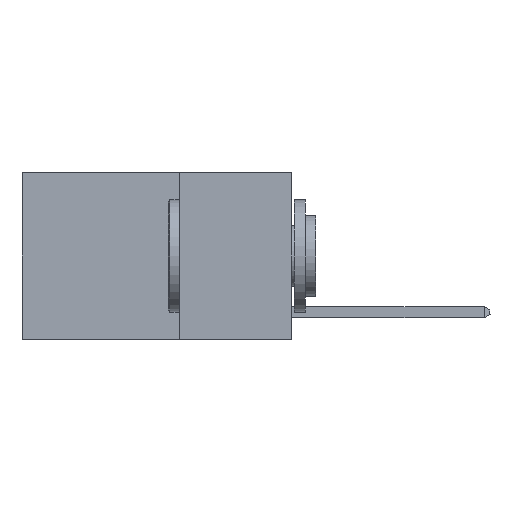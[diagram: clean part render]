
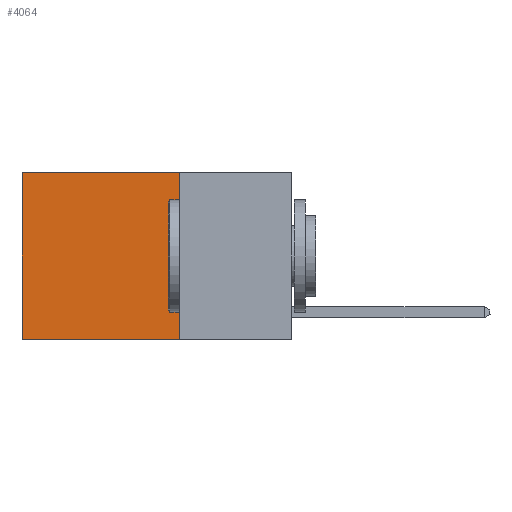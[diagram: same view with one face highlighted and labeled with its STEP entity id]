
A CAD part, left-side view. The second image highlights one B-rep face of the part: STEP entity #4064.
In plain terms, the highlighted planar face has unit normal (-1, 0, 0).
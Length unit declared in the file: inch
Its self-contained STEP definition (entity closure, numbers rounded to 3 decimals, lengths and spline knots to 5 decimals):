
#408 = AXIS2_PLACEMENT_3D ( 'NONE', #5421, #14235, #3438 ) ;
#579 = VECTOR ( 'NONE', #27081, 39.37008 ) ;
#3438 = DIRECTION ( 'NONE',  ( 0., 0., -1. ) ) ;
#3448 = CARTESIAN_POINT ( 'NONE',  ( 0.2625, 0.25, 0. ) ) ;
#3665 = EDGE_CURVE ( 'NONE', #5362, #18175, #24230, .T. ) ;
#4064 = ADVANCED_FACE ( 'NONE', ( #27777 ), #16918, .F. ) ;
#4445 = CARTESIAN_POINT ( 'NONE',  ( 0.2625, 0.25, 0. ) ) ;
#5362 = VERTEX_POINT ( 'NONE', #3448 ) ;
#5421 = CARTESIAN_POINT ( 'NONE',  ( 0.2625, 0.25, 0. ) ) ;
#7192 = ORIENTED_EDGE ( 'NONE', *, *, #16815, .T. ) ;
#8662 = DIRECTION ( 'NONE',  ( 0., 0., -1. ) ) ;
#9347 = CARTESIAN_POINT ( 'NONE',  ( 0.2625, 0.6, 0. ) ) ;
#9822 = LINE ( 'NONE', #24672, #24965 ) ;
#10295 = EDGE_CURVE ( 'NONE', #5362, #21108, #16379, .T. ) ;
#10707 = ORIENTED_EDGE ( 'NONE', *, *, #10295, .T. ) ;
#12171 = VECTOR ( 'NONE', #8662, 39.37008 ) ;
#13949 = CARTESIAN_POINT ( 'NONE',  ( 0.2625, 0.6, 0. ) ) ;
#14235 = DIRECTION ( 'NONE',  ( 1., 0., 0. ) ) ;
#15061 = EDGE_CURVE ( 'NONE', #18175, #23635, #9822, .T. ) ;
#16379 = LINE ( 'NONE', #20377, #21523 ) ;
#16815 = EDGE_CURVE ( 'NONE', #21108, #23635, #22817, .T. ) ;
#16918 = PLANE ( 'NONE',  #408 ) ;
#17274 = ORIENTED_EDGE ( 'NONE', *, *, #15061, .F. ) ;
#18175 = VERTEX_POINT ( 'NONE', #28071 ) ;
#18658 = DIRECTION ( 'NONE',  ( 0., 1., 0. ) ) ;
#18946 = ORIENTED_EDGE ( 'NONE', *, *, #3665, .F. ) ;
#20377 = CARTESIAN_POINT ( 'NONE',  ( 0.2625, 0.25, 0. ) ) ;
#20394 = DIRECTION ( 'NONE',  ( 0., 1., 0. ) ) ;
#21108 = VERTEX_POINT ( 'NONE', #9347 ) ;
#21523 = VECTOR ( 'NONE', #18658, 39.37008 ) ;
#22170 = EDGE_LOOP ( 'NONE', ( #7192, #17274, #18946, #10707 ) ) ;
#22817 = LINE ( 'NONE', #13949, #579 ) ;
#23635 = VERTEX_POINT ( 'NONE', #27673 ) ;
#24230 = LINE ( 'NONE', #4445, #12171 ) ;
#24672 = CARTESIAN_POINT ( 'NONE',  ( 0.2625, 0.25, -0.37 ) ) ;
#24965 = VECTOR ( 'NONE', #20394, 39.37008 ) ;
#27081 = DIRECTION ( 'NONE',  ( 0., 0., -1. ) ) ;
#27673 = CARTESIAN_POINT ( 'NONE',  ( 0.2625, 0.6, -0.37 ) ) ;
#27777 = FACE_OUTER_BOUND ( 'NONE', #22170, .T. ) ;
#28071 = CARTESIAN_POINT ( 'NONE',  ( 0.2625, 0.25, -0.37 ) ) ;
